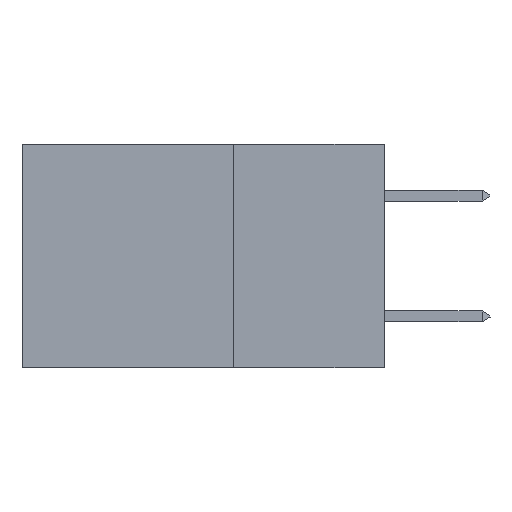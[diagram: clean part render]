
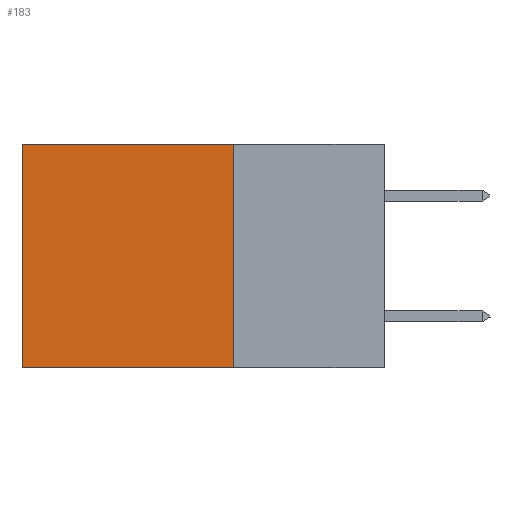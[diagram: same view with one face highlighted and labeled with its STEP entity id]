
A CAD part, left-side view. The second image highlights one B-rep face of the part: STEP entity #183.
In plain terms, the highlighted planar face has unit normal (-1, 0, 0).
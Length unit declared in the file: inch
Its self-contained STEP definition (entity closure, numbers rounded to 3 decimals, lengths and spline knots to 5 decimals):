
#183 = ADVANCED_FACE ( 'NONE', ( #13130 ), #16265, .F. ) ;
#277 = CARTESIAN_POINT ( 'NONE',  ( 0.2875, 0.25, -0.37 ) ) ;
#485 = DIRECTION ( 'NONE',  ( 0., 1., 0. ) ) ;
#556 = DIRECTION ( 'NONE',  ( 0., 0., -1. ) ) ;
#679 = CARTESIAN_POINT ( 'NONE',  ( 0.2875, 0.25, 0. ) ) ;
#1371 = EDGE_CURVE ( 'NONE', #10737, #19319, #3624, .T. ) ;
#1422 = DIRECTION ( 'NONE',  ( 0., 1., 0. ) ) ;
#1661 = ORIENTED_EDGE ( 'NONE', *, *, #18309, .T. ) ;
#3624 = LINE ( 'NONE', #16146, #8339 ) ;
#4883 = CARTESIAN_POINT ( 'NONE',  ( 0.2875, 0.6, 0. ) ) ;
#5126 = LINE ( 'NONE', #9161, #10077 ) ;
#7396 = ORIENTED_EDGE ( 'NONE', *, *, #16420, .F. ) ;
#8061 = LINE ( 'NONE', #14897, #9067 ) ;
#8339 = VECTOR ( 'NONE', #485, 39.37008 ) ;
#8904 = EDGE_CURVE ( 'NONE', #12666, #19234, #5126, .T. ) ;
#9067 = VECTOR ( 'NONE', #556, 39.37008 ) ;
#9161 = CARTESIAN_POINT ( 'NONE',  ( 0.2875, 0.25, -0.37 ) ) ;
#10077 = VECTOR ( 'NONE', #1422, 39.37008 ) ;
#10199 = ORIENTED_EDGE ( 'NONE', *, *, #1371, .T. ) ;
#10737 = VERTEX_POINT ( 'NONE', #15754 ) ;
#10872 = CARTESIAN_POINT ( 'NONE',  ( 0.2875, 0.6, -0.37 ) ) ;
#11266 = EDGE_LOOP ( 'NONE', ( #1661, #16657, #7396, #10199 ) ) ;
#11848 = VECTOR ( 'NONE', #15746, 39.37008 ) ;
#12666 = VERTEX_POINT ( 'NONE', #277 ) ;
#12856 = LINE ( 'NONE', #17344, #11848 ) ;
#13130 = FACE_OUTER_BOUND ( 'NONE', #11266, .T. ) ;
#14763 = AXIS2_PLACEMENT_3D ( 'NONE', #679, #15801, #19710 ) ;
#14897 = CARTESIAN_POINT ( 'NONE',  ( 0.2875, 0.6, 0. ) ) ;
#15746 = DIRECTION ( 'NONE',  ( 0., 0., -1. ) ) ;
#15754 = CARTESIAN_POINT ( 'NONE',  ( 0.2875, 0.25, 0. ) ) ;
#15801 = DIRECTION ( 'NONE',  ( 1., 0., 0. ) ) ;
#16146 = CARTESIAN_POINT ( 'NONE',  ( 0.2875, 0.25, 0. ) ) ;
#16265 = PLANE ( 'NONE',  #14763 ) ;
#16420 = EDGE_CURVE ( 'NONE', #10737, #12666, #12856, .T. ) ;
#16657 = ORIENTED_EDGE ( 'NONE', *, *, #8904, .F. ) ;
#17344 = CARTESIAN_POINT ( 'NONE',  ( 0.2875, 0.25, 0. ) ) ;
#18309 = EDGE_CURVE ( 'NONE', #19319, #19234, #8061, .T. ) ;
#19234 = VERTEX_POINT ( 'NONE', #10872 ) ;
#19319 = VERTEX_POINT ( 'NONE', #4883 ) ;
#19710 = DIRECTION ( 'NONE',  ( 0., 0., -1. ) ) ;
